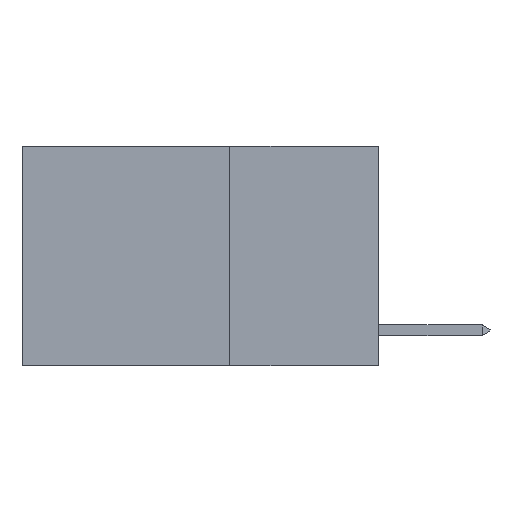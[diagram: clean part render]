
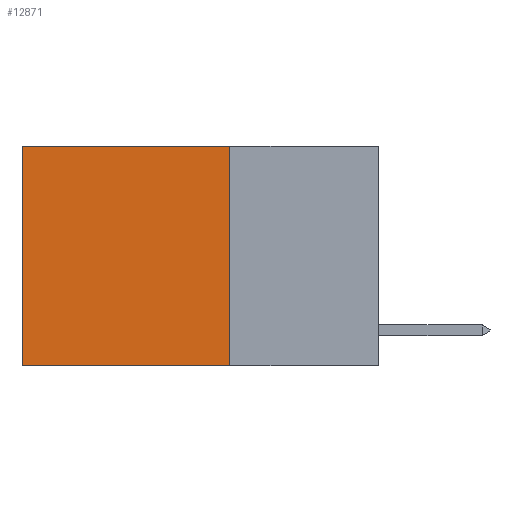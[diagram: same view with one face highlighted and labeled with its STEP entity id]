
A CAD part, left-side view. The second image highlights one B-rep face of the part: STEP entity #12871.
In plain terms, the highlighted planar face has unit normal (-1, 0, 0).
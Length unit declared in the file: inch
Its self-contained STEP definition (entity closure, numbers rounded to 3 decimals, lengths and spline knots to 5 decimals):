
#28 = ORIENTED_EDGE ( 'NONE', *, *, #10175, .F. ) ;
#65 = CARTESIAN_POINT ( 'NONE',  ( 0.2625, 0.25, 0. ) ) ;
#234 = VERTEX_POINT ( 'NONE', #13510 ) ;
#597 = EDGE_CURVE ( 'NONE', #234, #8832, #4513, .T. ) ;
#999 = DIRECTION ( 'NONE',  ( 0., 0., -1. ) ) ;
#1126 = CARTESIAN_POINT ( 'NONE',  ( 0.2625, 0.6, -0.37 ) ) ;
#1201 = DIRECTION ( 'NONE',  ( 0., 0., -1. ) ) ;
#1421 = ORIENTED_EDGE ( 'NONE', *, *, #6943, .T. ) ;
#2369 = EDGE_CURVE ( 'NONE', #11005, #5405, #4090, .T. ) ;
#2936 = CARTESIAN_POINT ( 'NONE',  ( 0.2625, 0.25, -0.37 ) ) ;
#3566 = ORIENTED_EDGE ( 'NONE', *, *, #2369, .T. ) ;
#4090 = LINE ( 'NONE', #10583, #13384 ) ;
#4513 = LINE ( 'NONE', #65, #9986 ) ;
#4592 = DIRECTION ( 'NONE',  ( 1., 0., 0. ) ) ;
#5374 = FACE_OUTER_BOUND ( 'NONE', #11566, .T. ) ;
#5393 = CARTESIAN_POINT ( 'NONE',  ( 0.2625, 0.25, -0.37 ) ) ;
#5405 = VERTEX_POINT ( 'NONE', #1126 ) ;
#5407 = DIRECTION ( 'NONE',  ( 0., 1., 0. ) ) ;
#6273 = CARTESIAN_POINT ( 'NONE',  ( 0.2625, 0.6, 0. ) ) ;
#6943 = EDGE_CURVE ( 'NONE', #234, #11005, #11568, .T. ) ;
#8512 = LINE ( 'NONE', #5393, #10103 ) ;
#8832 = VERTEX_POINT ( 'NONE', #2936 ) ;
#8898 = PLANE ( 'NONE',  #13317 ) ;
#9241 = ORIENTED_EDGE ( 'NONE', *, *, #597, .F. ) ;
#9986 = VECTOR ( 'NONE', #1201, 39.37008 ) ;
#10103 = VECTOR ( 'NONE', #12925, 39.37008 ) ;
#10175 = EDGE_CURVE ( 'NONE', #8832, #5405, #8512, .T. ) ;
#10583 = CARTESIAN_POINT ( 'NONE',  ( 0.2625, 0.6, 0. ) ) ;
#10881 = DIRECTION ( 'NONE',  ( 0., 0., -1. ) ) ;
#11005 = VERTEX_POINT ( 'NONE', #6273 ) ;
#11021 = CARTESIAN_POINT ( 'NONE',  ( 0.2625, 0.25, 0. ) ) ;
#11566 = EDGE_LOOP ( 'NONE', ( #3566, #28, #9241, #1421 ) ) ;
#11568 = LINE ( 'NONE', #13918, #12800 ) ;
#12800 = VECTOR ( 'NONE', #5407, 39.37008 ) ;
#12871 = ADVANCED_FACE ( 'NONE', ( #5374 ), #8898, .F. ) ;
#12925 = DIRECTION ( 'NONE',  ( 0., 1., 0. ) ) ;
#13317 = AXIS2_PLACEMENT_3D ( 'NONE', #11021, #4592, #10881 ) ;
#13384 = VECTOR ( 'NONE', #999, 39.37008 ) ;
#13510 = CARTESIAN_POINT ( 'NONE',  ( 0.2625, 0.25, 0. ) ) ;
#13918 = CARTESIAN_POINT ( 'NONE',  ( 0.2625, 0.25, 0. ) ) ;
